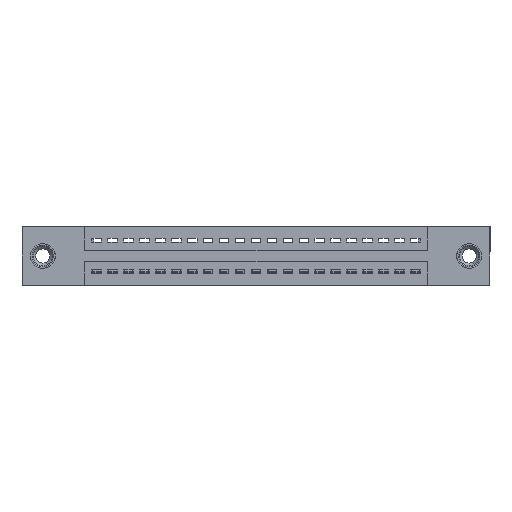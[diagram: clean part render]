
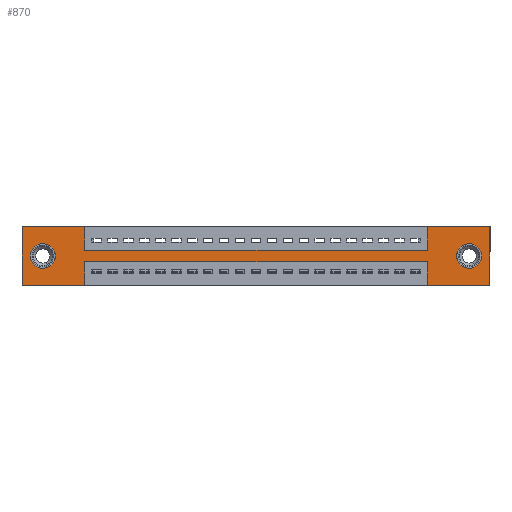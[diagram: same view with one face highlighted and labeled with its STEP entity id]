
A CAD part, front view. The second image highlights one B-rep face of the part: STEP entity #870.
In plain terms, the highlighted planar face has unit normal (0, -1, 0).
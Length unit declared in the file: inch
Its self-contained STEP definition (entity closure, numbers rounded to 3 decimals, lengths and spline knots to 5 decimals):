
#28 = ORIENTED_EDGE ( 'NONE', *, *, #8813, .F. ) ;
#29 = ORIENTED_EDGE ( 'NONE', *, *, #10632, .T. ) ;
#220 = EDGE_CURVE ( 'NONE', #10049, #7299, #14670, .T. ) ;
#312 = CARTESIAN_POINT ( 'NONE',  ( 0.3925, 0., -0.15 ) ) ;
#870 = ADVANCED_FACE ( 'NONE', ( #3138, #8146, #2672 ), #19109, .T. ) ;
#985 = VECTOR ( 'NONE', #3611, 39.37008 ) ;
#1361 = DIRECTION ( 'NONE',  ( 0., 0., -1. ) ) ;
#1459 = VERTEX_POINT ( 'NONE', #4765 ) ;
#1555 = ORIENTED_EDGE ( 'NONE', *, *, #16312, .F. ) ;
#1657 = ORIENTED_EDGE ( 'NONE', *, *, #1681, .F. ) ;
#1681 = EDGE_CURVE ( 'NONE', #7767, #16747, #19801, .T. ) ;
#1757 = CARTESIAN_POINT ( 'NONE',  ( 0., 0., -0.37 ) ) ;
#1900 = CARTESIAN_POINT ( 'NONE',  ( 2.935, 0., 0. ) ) ;
#1905 = ORIENTED_EDGE ( 'NONE', *, *, #11503, .F. ) ;
#1973 = DIRECTION ( 'NONE',  ( 0., 0., 1. ) ) ;
#2085 = DIRECTION ( 'NONE',  ( 0., 1., 0. ) ) ;
#2306 = AXIS2_PLACEMENT_3D ( 'NONE', #14587, #3283, #3496 ) ;
#2319 = CARTESIAN_POINT ( 'NONE',  ( 2.5425, 0., -0.22 ) ) ;
#2421 = ORIENTED_EDGE ( 'NONE', *, *, #2989, .F. ) ;
#2514 = EDGE_CURVE ( 'NONE', #14480, #7767, #13567, .T. ) ;
#2672 = FACE_OUTER_BOUND ( 'NONE', #17146, .T. ) ;
#2917 = ORIENTED_EDGE ( 'NONE', *, *, #11922, .F. ) ;
#2934 = VECTOR ( 'NONE', #5584, 39.37008 ) ;
#2989 = EDGE_CURVE ( 'NONE', #8242, #15762, #5912, .T. ) ;
#3077 = CARTESIAN_POINT ( 'NONE',  ( 0.3925, 0., -0.22 ) ) ;
#3138 = FACE_BOUND ( 'NONE', #10116, .T. ) ;
#3283 = DIRECTION ( 'NONE',  ( 0., 1., 0. ) ) ;
#3442 = AXIS2_PLACEMENT_3D ( 'NONE', #11653, #2085, #13231 ) ;
#3496 = DIRECTION ( 'NONE',  ( 0., 0., -1. ) ) ;
#3576 = CARTESIAN_POINT ( 'NONE',  ( 2.805, 0., -0.263 ) ) ;
#3611 = DIRECTION ( 'NONE',  ( 1., 0., 0. ) ) ;
#3648 = CARTESIAN_POINT ( 'NONE',  ( 0.3925, 0., 0. ) ) ;
#3664 = VERTEX_POINT ( 'NONE', #16056 ) ;
#3779 = CARTESIAN_POINT ( 'NONE',  ( 0.13, 0., -0.185 ) ) ;
#4707 = LINE ( 'NONE', #312, #985 ) ;
#4765 = CARTESIAN_POINT ( 'NONE',  ( 0.13, 0., -0.263 ) ) ;
#4769 = DIRECTION ( 'NONE',  ( 0., -1., 0. ) ) ;
#4867 = VECTOR ( 'NONE', #6844, 39.37008 ) ;
#4992 = DIRECTION ( 'NONE',  ( -1., 0., 0. ) ) ;
#5200 = VECTOR ( 'NONE', #11480, 39.37008 ) ;
#5284 = LINE ( 'NONE', #17519, #12064 ) ;
#5388 = CARTESIAN_POINT ( 'NONE',  ( 0., 0., 0. ) ) ;
#5546 = DIRECTION ( 'NONE',  ( 0., 0., -1. ) ) ;
#5584 = DIRECTION ( 'NONE',  ( 0., 0., 1. ) ) ;
#5680 = DIRECTION ( 'NONE',  ( 0., 1., 0. ) ) ;
#5732 = LINE ( 'NONE', #1900, #5200 ) ;
#5815 = VERTEX_POINT ( 'NONE', #14782 ) ;
#5912 = LINE ( 'NONE', #13033, #4867 ) ;
#5936 = CARTESIAN_POINT ( 'NONE',  ( 0.3925, 0., -0.37 ) ) ;
#5996 = EDGE_CURVE ( 'NONE', #5815, #13448, #8815, .T. ) ;
#6273 = CARTESIAN_POINT ( 'NONE',  ( 0., 0., 0. ) ) ;
#6386 = LINE ( 'NONE', #1757, #19587 ) ;
#6475 = ORIENTED_EDGE ( 'NONE', *, *, #9884, .T. ) ;
#6601 = CARTESIAN_POINT ( 'NONE',  ( 0.13, 0., -0.185 ) ) ;
#6695 = CARTESIAN_POINT ( 'NONE',  ( 2.5425, 0., -0.37 ) ) ;
#6844 = DIRECTION ( 'NONE',  ( 0., 0., 1. ) ) ;
#7250 = ORIENTED_EDGE ( 'NONE', *, *, #18560, .F. ) ;
#7299 = VERTEX_POINT ( 'NONE', #6695 ) ;
#7523 = EDGE_CURVE ( 'NONE', #16747, #8242, #4707, .T. ) ;
#7688 = EDGE_CURVE ( 'NONE', #7955, #14480, #9003, .T. ) ;
#7739 = AXIS2_PLACEMENT_3D ( 'NONE', #9602, #4769, #18978 ) ;
#7767 = VERTEX_POINT ( 'NONE', #3648 ) ;
#7955 = VERTEX_POINT ( 'NONE', #16516 ) ;
#7971 = DIRECTION ( 'NONE',  ( -1., 0., 0. ) ) ;
#8022 = CARTESIAN_POINT ( 'NONE',  ( 0.3925, 0., -0.37 ) ) ;
#8146 = FACE_BOUND ( 'NONE', #17313, .T. ) ;
#8242 = VERTEX_POINT ( 'NONE', #19303 ) ;
#8357 = CARTESIAN_POINT ( 'NONE',  ( 2.5425, 0., 0. ) ) ;
#8410 = DIRECTION ( 'NONE',  ( 1., 0., 0. ) ) ;
#8624 = VERTEX_POINT ( 'NONE', #2319 ) ;
#8813 = EDGE_CURVE ( 'NONE', #18713, #7955, #6386, .T. ) ;
#8815 = CIRCLE ( 'NONE', #2306, 0.078 ) ;
#8900 = CARTESIAN_POINT ( 'NONE',  ( 0.3925, 0., 0. ) ) ;
#9003 = LINE ( 'NONE', #19421, #10726 ) ;
#9582 = CARTESIAN_POINT ( 'NONE',  ( 0.3925, 0., -0.15 ) ) ;
#9602 = CARTESIAN_POINT ( 'NONE',  ( 0., 0., -0.37 ) ) ;
#9841 = CARTESIAN_POINT ( 'NONE',  ( 2.935, 0., 0. ) ) ;
#9884 = EDGE_CURVE ( 'NONE', #1459, #3664, #16446, .T. ) ;
#9943 = VECTOR ( 'NONE', #4992, 39.37008 ) ;
#10049 = VERTEX_POINT ( 'NONE', #17557 ) ;
#10085 = VERTEX_POINT ( 'NONE', #9841 ) ;
#10116 = EDGE_LOOP ( 'NONE', ( #18620, #10702 ) ) ;
#10190 = LINE ( 'NONE', #14990, #2934 ) ;
#10403 = LINE ( 'NONE', #13261, #18814 ) ;
#10484 = DIRECTION ( 'NONE',  ( 0., 0., 1. ) ) ;
#10551 = EDGE_CURVE ( 'NONE', #7299, #8624, #10190, .T. ) ;
#10632 = EDGE_CURVE ( 'NONE', #3664, #1459, #16137, .T. ) ;
#10702 = ORIENTED_EDGE ( 'NONE', *, *, #12416, .T. ) ;
#10726 = VECTOR ( 'NONE', #1973, 39.37008 ) ;
#11480 = DIRECTION ( 'NONE',  ( 0., 0., -1. ) ) ;
#11503 = EDGE_CURVE ( 'NONE', #15762, #10085, #10403, .T. ) ;
#11653 = CARTESIAN_POINT ( 'NONE',  ( 2.805, 0., -0.185 ) ) ;
#11922 = EDGE_CURVE ( 'NONE', #13559, #18713, #16068, .T. ) ;
#12064 = VECTOR ( 'NONE', #7971, 39.37008 ) ;
#12416 = EDGE_CURVE ( 'NONE', #13448, #5815, #13328, .T. ) ;
#12855 = ORIENTED_EDGE ( 'NONE', *, *, #2514, .F. ) ;
#13033 = CARTESIAN_POINT ( 'NONE',  ( 2.5425, 0., 0. ) ) ;
#13231 = DIRECTION ( 'NONE',  ( 0., 0., -1. ) ) ;
#13261 = CARTESIAN_POINT ( 'NONE',  ( 0., 0., 0. ) ) ;
#13328 = CIRCLE ( 'NONE', #3442, 0.078 ) ;
#13448 = VERTEX_POINT ( 'NONE', #3576 ) ;
#13559 = VERTEX_POINT ( 'NONE', #3077 ) ;
#13567 = LINE ( 'NONE', #5388, #14293 ) ;
#13794 = DIRECTION ( 'NONE',  ( 0., 0., 1. ) ) ;
#14293 = VECTOR ( 'NONE', #18277, 39.37008 ) ;
#14480 = VERTEX_POINT ( 'NONE', #6273 ) ;
#14482 = CARTESIAN_POINT ( 'NONE',  ( 0., 0., -0.37 ) ) ;
#14487 = AXIS2_PLACEMENT_3D ( 'NONE', #6601, #20078, #10484 ) ;
#14587 = CARTESIAN_POINT ( 'NONE',  ( 2.805, 0., -0.185 ) ) ;
#14670 = LINE ( 'NONE', #14482, #9943 ) ;
#14782 = CARTESIAN_POINT ( 'NONE',  ( 2.805, 0., -0.107 ) ) ;
#14990 = CARTESIAN_POINT ( 'NONE',  ( 2.5425, 0., -0.37 ) ) ;
#15666 = ORIENTED_EDGE ( 'NONE', *, *, #220, .F. ) ;
#15762 = VERTEX_POINT ( 'NONE', #8357 ) ;
#15899 = ORIENTED_EDGE ( 'NONE', *, *, #7688, .F. ) ;
#15960 = ORIENTED_EDGE ( 'NONE', *, *, #7523, .F. ) ;
#16056 = CARTESIAN_POINT ( 'NONE',  ( 0.13, 0., -0.107 ) ) ;
#16068 = LINE ( 'NONE', #5936, #16830 ) ;
#16137 = CIRCLE ( 'NONE', #14487, 0.078 ) ;
#16312 = EDGE_CURVE ( 'NONE', #8624, #13559, #5284, .T. ) ;
#16446 = CIRCLE ( 'NONE', #16495, 0.078 ) ;
#16495 = AXIS2_PLACEMENT_3D ( 'NONE', #3779, #5680, #13794 ) ;
#16516 = CARTESIAN_POINT ( 'NONE',  ( 0., 0., -0.37 ) ) ;
#16747 = VERTEX_POINT ( 'NONE', #9582 ) ;
#16830 = VECTOR ( 'NONE', #1361, 39.37008 ) ;
#17146 = EDGE_LOOP ( 'NONE', ( #2917, #1555, #18768, #15666, #7250, #1905, #2421, #15960, #1657, #12855, #15899, #28 ) ) ;
#17313 = EDGE_LOOP ( 'NONE', ( #29, #6475 ) ) ;
#17519 = CARTESIAN_POINT ( 'NONE',  ( 0.3925, 0., -0.22 ) ) ;
#17557 = CARTESIAN_POINT ( 'NONE',  ( 2.935, 0., -0.37 ) ) ;
#17577 = VECTOR ( 'NONE', #5546, 39.37008 ) ;
#18277 = DIRECTION ( 'NONE',  ( 1., 0., 0. ) ) ;
#18560 = EDGE_CURVE ( 'NONE', #10085, #10049, #5732, .T. ) ;
#18620 = ORIENTED_EDGE ( 'NONE', *, *, #5996, .T. ) ;
#18713 = VERTEX_POINT ( 'NONE', #8022 ) ;
#18768 = ORIENTED_EDGE ( 'NONE', *, *, #10551, .F. ) ;
#18814 = VECTOR ( 'NONE', #8410, 39.37008 ) ;
#18978 = DIRECTION ( 'NONE',  ( 0., 0., -1. ) ) ;
#19109 = PLANE ( 'NONE',  #7739 ) ;
#19303 = CARTESIAN_POINT ( 'NONE',  ( 2.5425, 0., -0.15 ) ) ;
#19421 = CARTESIAN_POINT ( 'NONE',  ( 0., 0., 0. ) ) ;
#19587 = VECTOR ( 'NONE', #20599, 39.37008 ) ;
#19801 = LINE ( 'NONE', #8900, #17577 ) ;
#20078 = DIRECTION ( 'NONE',  ( 0., 1., 0. ) ) ;
#20599 = DIRECTION ( 'NONE',  ( -1., 0., 0. ) ) ;
